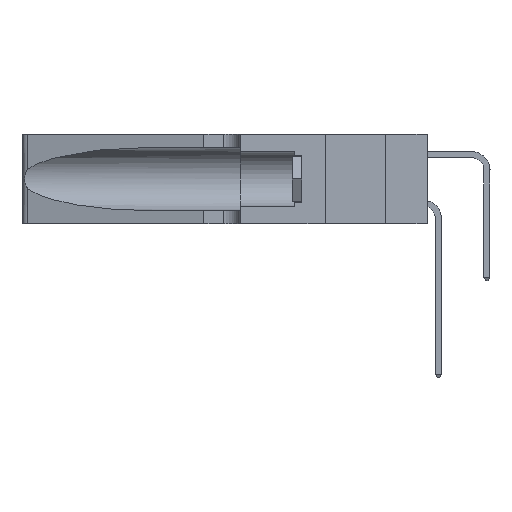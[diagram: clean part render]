
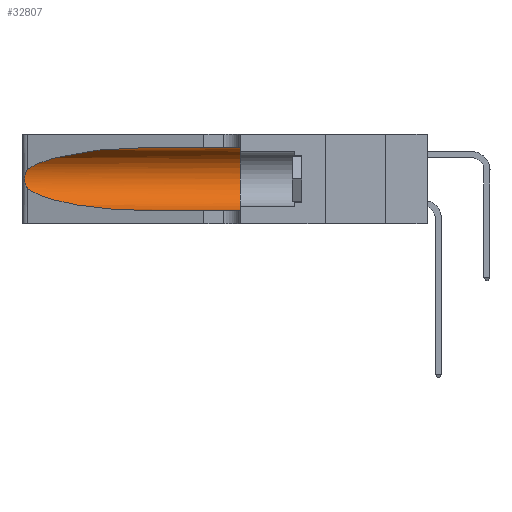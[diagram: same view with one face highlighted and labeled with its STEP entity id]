
A CAD part, left-side view. The second image highlights one B-rep face of the part: STEP entity #32807.
In plain terms, the highlighted cylindrical face has radius 3.308 mm (diameter 6.617 mm), a partial arc.
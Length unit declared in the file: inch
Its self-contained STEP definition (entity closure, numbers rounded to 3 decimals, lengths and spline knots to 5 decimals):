
#50 = DIRECTION ( 'NONE',  ( 0., 0., -1. ) ) ;
#2177 = CARTESIAN_POINT ( 'NONE',  ( 0.1305, 0.35, 0.185 ) ) ;
#2460 = EDGE_CURVE ( 'NONE', #22854, #30554, #15269, .T. ) ;
#2839 = CARTESIAN_POINT ( 'NONE',  ( 0.26075, 1.23896, 0.19203 ) ) ;
#3662 = CARTESIAN_POINT ( 'NONE',  ( 0.18966, 0.96281, 0.31525 ) ) ;
#3712 = AXIS2_PLACEMENT_3D ( 'NONE', #2177, #30709, #25155 ) ;
#4262 = CARTESIAN_POINT ( 'NONE',  ( 0.25639, 1.23186, 0.15144 ) ) ;
#6451 = CARTESIAN_POINT ( 'NONE',  ( 0.25487, 1.22718, 0.14631 ) ) ;
#7330 = CARTESIAN_POINT ( 'NONE',  ( 0.1305, 0.35, 0.31525 ) ) ;
#7833 = VECTOR ( 'NONE', #33193, 39.37008 ) ;
#8702 = EDGE_LOOP ( 'NONE', ( #27618, #25326, #22577, #12948, #30861, #31491 ) ) ;
#8705 = DIRECTION ( 'NONE',  ( 0., -1., 0. ) ) ;
#9703 = VECTOR ( 'NONE', #14337, 39.37008 ) ;
#9741 = CARTESIAN_POINT ( 'NONE',  ( 0.25487, 1.22718, 0.22369 ) ) ;
#9972 = CARTESIAN_POINT ( 'NONE',  ( 0.18966, 0.96281, 0.05475 ) ) ;
#10183 = CARTESIAN_POINT ( 'NONE',  ( 0.25487, 1.22718, 0.22369 ) ) ;
#12702 = LINE ( 'NONE', #19101, #7833 ) ;
#12948 = ORIENTED_EDGE ( 'NONE', *, *, #19031, .T. ) ;
#14191 =( BOUNDED_CURVE ( )  B_SPLINE_CURVE ( 3, ( #35239, #3662, #34987, #9741 ),
 .UNSPECIFIED., .F., .T. ) 
 B_SPLINE_CURVE_WITH_KNOTS ( ( 4, 4 ),
 ( 1.5708, 2.84003 ),
 .UNSPECIFIED. ) 
 CURVE ( )  GEOMETRIC_REPRESENTATION_ITEM ( )  RATIONAL_B_SPLINE_CURVE ( ( 1., 0.87, 0.87, 1. ) ) 
 REPRESENTATION_ITEM ( '' )  );
#14253 = CARTESIAN_POINT ( 'NONE',  ( 0.1305, 0.72297, 0.31525 ) ) ;
#14337 = DIRECTION ( 'NONE',  ( 0., -1., 0. ) ) ;
#14559 = VERTEX_POINT ( 'NONE', #14253 ) ;
#14986 = CARTESIAN_POINT ( 'NONE',  ( 0.26075, 1.23896, 0.178 ) ) ;
#15269 = B_SPLINE_CURVE_WITH_KNOTS ( 'NONE', 3,
 ( #10183, #24604, #15797, #30281, #18689, #33169, #2839, #14986, #17450, #22162, #17347, #4262, #25126, #20042 ),
 .UNSPECIFIED., .F., .F.,
 ( 4, 2, 2, 2, 2, 2, 4 ),
 ( 0., 0.00027, 0.00053, 0.00107, 0.0016, 0.00187, 0.00214 ),
 .UNSPECIFIED. ) ;
#15797 = CARTESIAN_POINT ( 'NONE',  ( 0.25639, 1.23184, 0.21858 ) ) ;
#16922 = EDGE_CURVE ( 'NONE', #14559, #32593, #12702, .T. ) ;
#17347 = CARTESIAN_POINT ( 'NONE',  ( 0.25789, 1.23486, 0.15765 ) ) ;
#17450 = CARTESIAN_POINT ( 'NONE',  ( 0.26017, 1.23833, 0.17102 ) ) ;
#17706 = FACE_OUTER_BOUND ( 'NONE', #8702, .T. ) ;
#18331 = EDGE_CURVE ( 'NONE', #30554, #24779, #32942, .T. ) ;
#18689 = CARTESIAN_POINT ( 'NONE',  ( 0.25854, 1.2359, 0.20912 ) ) ;
#19031 = EDGE_CURVE ( 'NONE', #24779, #34339, #29811, .T. ) ;
#19101 = CARTESIAN_POINT ( 'NONE',  ( 0.1305, 1.61858, 0.31525 ) ) ;
#20042 = CARTESIAN_POINT ( 'NONE',  ( 0.25487, 1.22718, 0.14631 ) ) ;
#20218 = CARTESIAN_POINT ( 'NONE',  ( 0.1305, 0.72297, 0.05475 ) ) ;
#22162 = CARTESIAN_POINT ( 'NONE',  ( 0.25856, 1.23593, 0.16098 ) ) ;
#22577 = ORIENTED_EDGE ( 'NONE', *, *, #18331, .T. ) ;
#22854 = VERTEX_POINT ( 'NONE', #33497 ) ;
#22856 = EDGE_CURVE ( 'NONE', #32593, #34339, #26896, .T. ) ;
#24604 = CARTESIAN_POINT ( 'NONE',  ( 0.25555, 1.22994, 0.2215 ) ) ;
#24779 = VERTEX_POINT ( 'NONE', #20218 ) ;
#25126 = CARTESIAN_POINT ( 'NONE',  ( 0.25555, 1.22993, 0.14849 ) ) ;
#25155 = DIRECTION ( 'NONE',  ( 0., 0., 1. ) ) ;
#25326 = ORIENTED_EDGE ( 'NONE', *, *, #2460, .T. ) ;
#26896 = CIRCLE ( 'NONE', #3712, 0.13025 ) ;
#26992 = CARTESIAN_POINT ( 'NONE',  ( 0.1305, 0.72297, 0.05475 ) ) ;
#27122 = CARTESIAN_POINT ( 'NONE',  ( 0.2373, 1.15595, 0.08982 ) ) ;
#27157 = AXIS2_PLACEMENT_3D ( 'NONE', #28928, #8705, #50 ) ;
#27618 = ORIENTED_EDGE ( 'NONE', *, *, #33652, .T. ) ;
#28928 = CARTESIAN_POINT ( 'NONE',  ( 0.1305, 1.61858, 0.185 ) ) ;
#29811 = LINE ( 'NONE', #30944, #9703 ) ;
#30281 = CARTESIAN_POINT ( 'NONE',  ( 0.25787, 1.23484, 0.2124 ) ) ;
#30554 = VERTEX_POINT ( 'NONE', #6451 ) ;
#30709 = DIRECTION ( 'NONE',  ( 0., 1., 0. ) ) ;
#30861 = ORIENTED_EDGE ( 'NONE', *, *, #22856, .F. ) ;
#30944 = CARTESIAN_POINT ( 'NONE',  ( 0.1305, 1.61858, 0.05475 ) ) ;
#31491 = ORIENTED_EDGE ( 'NONE', *, *, #16922, .F. ) ;
#31927 = CARTESIAN_POINT ( 'NONE',  ( 0.1305, 0.35, 0.05475 ) ) ;
#32593 = VERTEX_POINT ( 'NONE', #7330 ) ;
#32680 = CARTESIAN_POINT ( 'NONE',  ( 0.25487, 1.22718, 0.14631 ) ) ;
#32807 = ADVANCED_FACE ( 'NONE', ( #17706 ), #35586, .F. ) ;
#32942 =( BOUNDED_CURVE ( )  B_SPLINE_CURVE ( 3, ( #32680, #27122, #9972, #26992 ),
 .UNSPECIFIED., .F., .T. ) 
 B_SPLINE_CURVE_WITH_KNOTS ( ( 4, 4 ),
 ( 3.44316, 4.71239 ),
 .UNSPECIFIED. ) 
 CURVE ( )  GEOMETRIC_REPRESENTATION_ITEM ( )  RATIONAL_B_SPLINE_CURVE ( ( 1., 0.87, 0.87, 1. ) ) 
 REPRESENTATION_ITEM ( '' )  );
#33169 = CARTESIAN_POINT ( 'NONE',  ( 0.26018, 1.23835, 0.19895 ) ) ;
#33193 = DIRECTION ( 'NONE',  ( 0., -1., 0. ) ) ;
#33497 = CARTESIAN_POINT ( 'NONE',  ( 0.25487, 1.22718, 0.22369 ) ) ;
#33652 = EDGE_CURVE ( 'NONE', #14559, #22854, #14191, .T. ) ;
#34339 = VERTEX_POINT ( 'NONE', #31927 ) ;
#34987 = CARTESIAN_POINT ( 'NONE',  ( 0.2373, 1.15595, 0.28018 ) ) ;
#35239 = CARTESIAN_POINT ( 'NONE',  ( 0.1305, 0.72297, 0.31525 ) ) ;
#35586 = CYLINDRICAL_SURFACE ( 'NONE', #27157, 0.13025 ) ;
